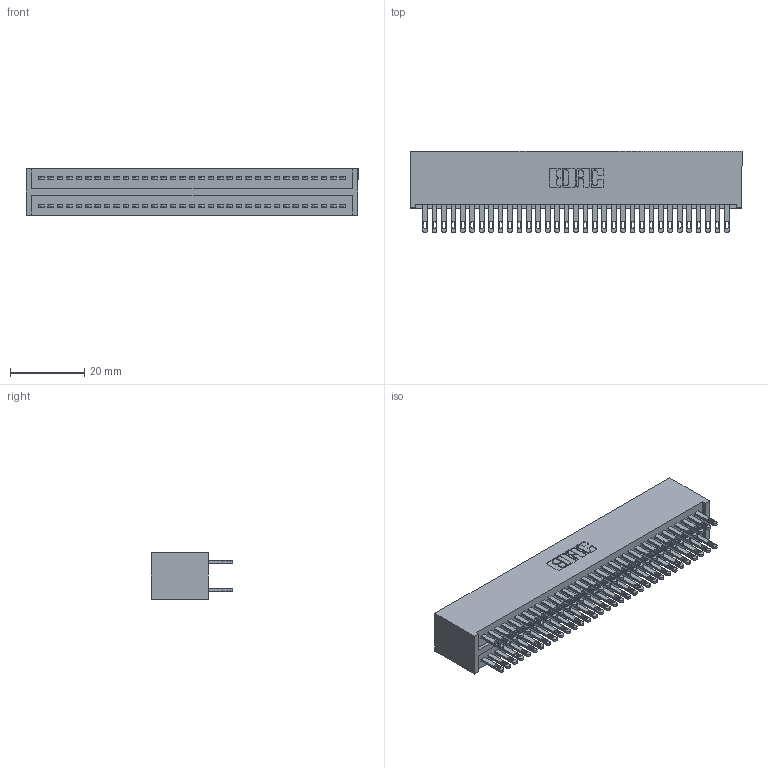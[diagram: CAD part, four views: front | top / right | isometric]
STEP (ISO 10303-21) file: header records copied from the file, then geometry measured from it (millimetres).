
FILE_DESCRIPTION (( 'STEP AP203' ), '1' );
FILE_NAME ('325-066-500-201.STEP', '2020-02-25T03:15:48', ( '' ), ( '' ), 'SwSTEP 2.0', 'SolidWorks 2016', '' );
FILE_SCHEMA (( 'CONFIG_CONTROL_DESIGN' ));
Length unit declared in the file: inch
Products named in the file (3): 325-292-001_325-293-100; 325 Part_Lugless; 325-066-500-201
Assembly tree (67 placements, depth 2):
  325-066-500-201
    325 Part_Lugless
    325-292-001_325-293-100  x66
Bounding box: 89.46 x 21.84 x 12.45 mm (x, y, z)
Volume: 12275.8 mm3; surface area: 15996 mm2
Topology: 67 solids, 67 shells, 3274 faces, 9989 edges, 6658 vertices
Faces by surface type: plane 2046, cylinder 1228
Entity records: 22047 total; most frequent: CARTESIAN_POINT 3662, ORIENTED_EDGE 3598, DIRECTION 3139, EDGE_CURVE 1799, LINE 1675, VECTOR 1675, VERTEX_POINT 1198, AXIS2_PLACEMENT_3D 732
